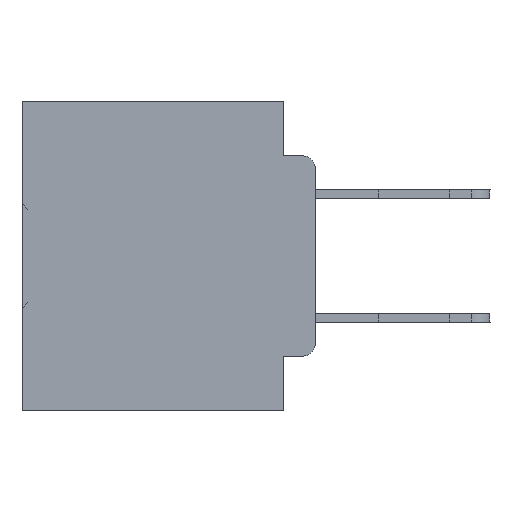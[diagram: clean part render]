
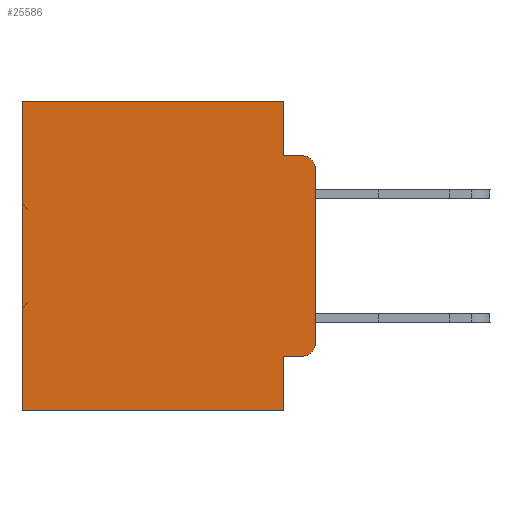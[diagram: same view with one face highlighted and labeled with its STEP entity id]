
A CAD part, left-side view. The second image highlights one B-rep face of the part: STEP entity #25586.
In plain terms, the highlighted planar face has unit normal (-1, 0, 0).
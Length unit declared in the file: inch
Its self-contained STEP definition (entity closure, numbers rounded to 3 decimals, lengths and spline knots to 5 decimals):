
#827 = EDGE_CURVE ( 'NONE', #28915, #30273, #12598, .T. ) ;
#1081 = CARTESIAN_POINT ( 'NONE',  ( 0.298, 0., 0. ) ) ;
#1614 = DIRECTION ( 'NONE',  ( 0., 0., -1. ) ) ;
#1667 = EDGE_CURVE ( 'NONE', #4345, #10130, #23107, .T. ) ;
#1822 = CARTESIAN_POINT ( 'NONE',  ( 0.298, 0.051, 0. ) ) ;
#2573 = LINE ( 'NONE', #28743, #28271 ) ;
#2706 = CARTESIAN_POINT ( 'NONE',  ( 0.298, 0.051, -0.4115 ) ) ;
#3268 = AXIS2_PLACEMENT_3D ( 'NONE', #10506, #21836, #7368 ) ;
#3822 = DIRECTION ( 'NONE',  ( 0., 0., -1. ) ) ;
#4345 = VERTEX_POINT ( 'NONE', #32157 ) ;
#4353 = LINE ( 'NONE', #28943, #28572 ) ;
#4403 = CARTESIAN_POINT ( 'NONE',  ( 0.298, 0.473, 0. ) ) ;
#5115 = DIRECTION ( 'NONE',  ( -1., 0., 0. ) ) ;
#5601 = AXIS2_PLACEMENT_3D ( 'NONE', #10606, #19386, #1614 ) ;
#6210 = AXIS2_PLACEMENT_3D ( 'NONE', #34633, #5115, #11007 ) ;
#6774 = EDGE_CURVE ( 'NONE', #28915, #13858, #32780, .T. ) ;
#6947 = DIRECTION ( 'NONE',  ( 0., 1., 0. ) ) ;
#7368 = DIRECTION ( 'NONE',  ( 0., 0., -1. ) ) ;
#7890 = CARTESIAN_POINT ( 'NONE',  ( 0.298, 0.051, -0.4115 ) ) ;
#7901 = DIRECTION ( 'NONE',  ( 0., 0., -1. ) ) ;
#7911 = EDGE_CURVE ( 'NONE', #34354, #19045, #4353, .T. ) ;
#9226 = EDGE_CURVE ( 'NONE', #33298, #11937, #26790, .T. ) ;
#9322 = EDGE_CURVE ( 'NONE', #13858, #38534, #24946, .T. ) ;
#9742 = PLANE ( 'NONE',  #3268 ) ;
#10130 = VERTEX_POINT ( 'NONE', #33475 ) ;
#10506 = CARTESIAN_POINT ( 'NONE',  ( 0.298, 0., 0. ) ) ;
#10606 = CARTESIAN_POINT ( 'NONE',  ( 0.298, 0.02, -0.3915 ) ) ;
#10678 = DIRECTION ( 'NONE',  ( 0., 1., 0. ) ) ;
#11007 = DIRECTION ( 'NONE',  ( 0., 0., -1. ) ) ;
#11018 = EDGE_CURVE ( 'NONE', #30273, #19045, #15363, .T. ) ;
#11450 = LINE ( 'NONE', #13599, #19700 ) ;
#11937 = VERTEX_POINT ( 'NONE', #15018 ) ;
#12412 = DIRECTION ( 'NONE',  ( 0., 0., -1. ) ) ;
#12598 = LINE ( 'NONE', #21219, #15639 ) ;
#12608 = CARTESIAN_POINT ( 'NONE',  ( 0.298, 0., -0.5 ) ) ;
#13599 = CARTESIAN_POINT ( 'NONE',  ( 0.298, 0., 0. ) ) ;
#13858 = VERTEX_POINT ( 'NONE', #25939 ) ;
#15018 = CARTESIAN_POINT ( 'NONE',  ( 0.298, 0.02, -0.0885 ) ) ;
#15363 = LINE ( 'NONE', #12608, #21492 ) ;
#15639 = VECTOR ( 'NONE', #12412, 39.37008 ) ;
#16114 = LINE ( 'NONE', #1081, #37048 ) ;
#17046 = ORIENTED_EDGE ( 'NONE', *, *, #33178, .F. ) ;
#19045 = VERTEX_POINT ( 'NONE', #26938 ) ;
#19386 = DIRECTION ( 'NONE',  ( -1., 0., 0. ) ) ;
#19700 = VECTOR ( 'NONE', #10678, 39.37008 ) ;
#19816 = ORIENTED_EDGE ( 'NONE', *, *, #6774, .T. ) ;
#20397 = ORIENTED_EDGE ( 'NONE', *, *, #9226, .T. ) ;
#21097 = EDGE_CURVE ( 'NONE', #4345, #34354, #11450, .T. ) ;
#21219 = CARTESIAN_POINT ( 'NONE',  ( 0.298, 0.051, 0. ) ) ;
#21345 = ORIENTED_EDGE ( 'NONE', *, *, #1667, .F. ) ;
#21439 = ORIENTED_EDGE ( 'NONE', *, *, #7911, .T. ) ;
#21492 = VECTOR ( 'NONE', #6947, 39.37008 ) ;
#21836 = DIRECTION ( 'NONE',  ( 1., 0., 0. ) ) ;
#22946 = ORIENTED_EDGE ( 'NONE', *, *, #21097, .T. ) ;
#23107 = LINE ( 'NONE', #1822, #29911 ) ;
#24946 = CIRCLE ( 'NONE', #5601, 0.02 ) ;
#25432 = DIRECTION ( 'NONE',  ( 0., 0., -1. ) ) ;
#25586 = ADVANCED_FACE ( 'NONE', ( #27892 ), #9742, .F. ) ;
#25939 = CARTESIAN_POINT ( 'NONE',  ( 0.298, 0.02, -0.4115 ) ) ;
#26396 = DIRECTION ( 'NONE',  ( 0., -1., 0. ) ) ;
#26790 = CIRCLE ( 'NONE', #6210, 0.02 ) ;
#26938 = CARTESIAN_POINT ( 'NONE',  ( 0.298, 0.473, -0.5 ) ) ;
#27892 = FACE_OUTER_BOUND ( 'NONE', #29265, .T. ) ;
#28271 = VECTOR ( 'NONE', #26396, 39.37008 ) ;
#28572 = VECTOR ( 'NONE', #25432, 39.37008 ) ;
#28743 = CARTESIAN_POINT ( 'NONE',  ( 0.298, 0.051, -0.0885 ) ) ;
#28915 = VERTEX_POINT ( 'NONE', #7890 ) ;
#28943 = CARTESIAN_POINT ( 'NONE',  ( 0.298, 0.473, 0. ) ) ;
#29000 = ORIENTED_EDGE ( 'NONE', *, *, #32966, .F. ) ;
#29265 = EDGE_LOOP ( 'NONE', ( #29000, #20397, #17046, #21345, #22946, #21439, #31326, #37070, #19816, #33542 ) ) ;
#29655 = DIRECTION ( 'NONE',  ( 0., -1., 0. ) ) ;
#29911 = VECTOR ( 'NONE', #7901, 39.37008 ) ;
#30273 = VERTEX_POINT ( 'NONE', #33927 ) ;
#30411 = CARTESIAN_POINT ( 'NONE',  ( 0.298, 0., -0.3915 ) ) ;
#31326 = ORIENTED_EDGE ( 'NONE', *, *, #11018, .F. ) ;
#32157 = CARTESIAN_POINT ( 'NONE',  ( 0.298, 0.051, 0. ) ) ;
#32780 = LINE ( 'NONE', #2706, #35053 ) ;
#32966 = EDGE_CURVE ( 'NONE', #33298, #38534, #16114, .T. ) ;
#33178 = EDGE_CURVE ( 'NONE', #10130, #11937, #2573, .T. ) ;
#33298 = VERTEX_POINT ( 'NONE', #36168 ) ;
#33475 = CARTESIAN_POINT ( 'NONE',  ( 0.298, 0.051, -0.0885 ) ) ;
#33542 = ORIENTED_EDGE ( 'NONE', *, *, #9322, .T. ) ;
#33927 = CARTESIAN_POINT ( 'NONE',  ( 0.298, 0.051, -0.5 ) ) ;
#34354 = VERTEX_POINT ( 'NONE', #4403 ) ;
#34633 = CARTESIAN_POINT ( 'NONE',  ( 0.298, 0.02, -0.1085 ) ) ;
#35053 = VECTOR ( 'NONE', #29655, 39.37008 ) ;
#36168 = CARTESIAN_POINT ( 'NONE',  ( 0.298, 0., -0.1085 ) ) ;
#37048 = VECTOR ( 'NONE', #3822, 39.37008 ) ;
#37070 = ORIENTED_EDGE ( 'NONE', *, *, #827, .F. ) ;
#38534 = VERTEX_POINT ( 'NONE', #30411 ) ;
